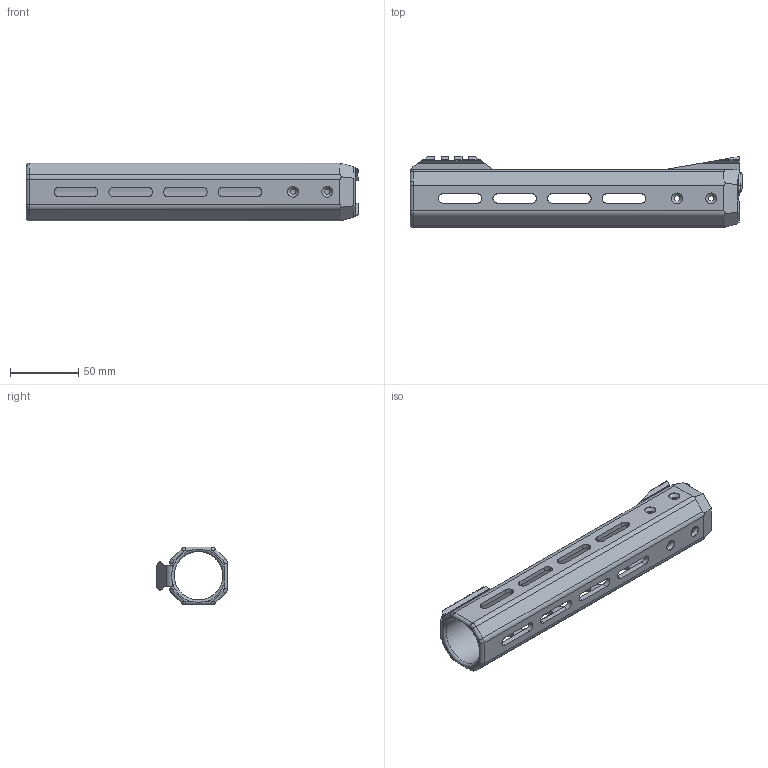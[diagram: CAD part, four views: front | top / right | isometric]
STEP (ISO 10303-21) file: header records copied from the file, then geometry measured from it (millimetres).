
FILE_DESCRIPTION(/* description */ (''),/* implementation_level */ '2;1');
FILE_NAME(/* name */ 'Shroud.step',/* time_stamp */ '2020-11-25T01:28:50-05:00',/* author */ (''),/* organization */ (''),/* preprocessor_version */ 'ST-DEVELOPER v18.1',/* originating_system */ 'Autodesk Translation Framework v9.3.0.1241',/* authorisation */ '');
FILE_SCHEMA (('AUTOMOTIVE_DESIGN { 1 0 10303 214 3 1 1 }'));
Length unit declared in the file: millimetre
Products named in the file (1): Shroud
Bounding box: 243.3 x 52.03 x 42.5 mm (x, y, z)
Volume: 146710.3 mm3; surface area: 63271.3 mm2
Topology: 1 solids, 1 shells, 199 faces, 553 edges, 354 vertices
Faces by surface type: plane 117, cylinder 67, bspline 8, cone 6, torus 1
Full cylindrical faces by diameter (mm): 4 x6, 8 x6, 35.542 x1
Entity records: 7060 total; most frequent: CARTESIAN_POINT 1878, ORIENTED_EDGE 1106, DIRECTION 1020, EDGE_CURVE 553, LINE 378, VECTOR 378, VERTEX_POINT 354, AXIS2_PLACEMENT_3D 321
